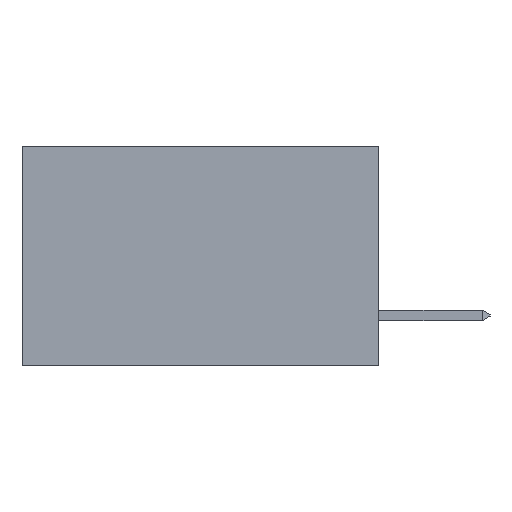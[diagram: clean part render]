
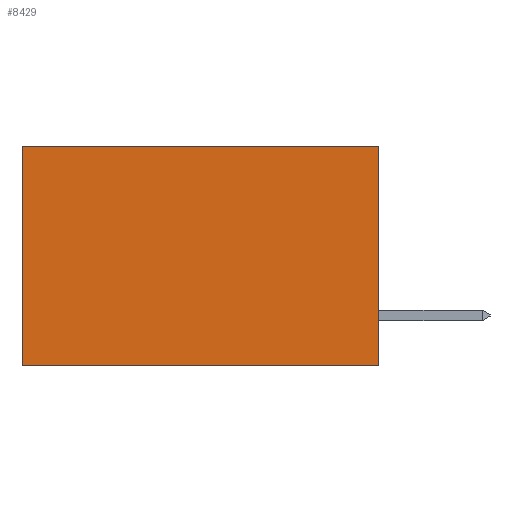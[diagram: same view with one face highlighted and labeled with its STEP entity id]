
A CAD part, left-side view. The second image highlights one B-rep face of the part: STEP entity #8429.
In plain terms, the highlighted planar face has unit normal (-1, 0, 0).
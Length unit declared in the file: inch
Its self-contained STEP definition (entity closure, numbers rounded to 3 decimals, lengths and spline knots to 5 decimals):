
#225 = PLANE ( 'NONE',  #2676 ) ;
#362 = CARTESIAN_POINT ( 'NONE',  ( 0.298, 0., 0. ) ) ;
#489 = CARTESIAN_POINT ( 'NONE',  ( 0.298, 0.6, 0. ) ) ;
#917 = VERTEX_POINT ( 'NONE', #10837 ) ;
#1516 = ORIENTED_EDGE ( 'NONE', *, *, #3124, .F. ) ;
#2676 = AXIS2_PLACEMENT_3D ( 'NONE', #362, #3206, #3161 ) ;
#2751 = CARTESIAN_POINT ( 'NONE',  ( 0.298, 0., 0. ) ) ;
#3083 = EDGE_CURVE ( 'NONE', #8026, #4044, #15981, .T. ) ;
#3124 = EDGE_CURVE ( 'NONE', #3225, #917, #15474, .T. ) ;
#3145 = LINE ( 'NONE', #2751, #19658 ) ;
#3161 = DIRECTION ( 'NONE',  ( 0., 0., -1. ) ) ;
#3206 = DIRECTION ( 'NONE',  ( 1., 0., 0. ) ) ;
#3225 = VERTEX_POINT ( 'NONE', #13918 ) ;
#3390 = ORIENTED_EDGE ( 'NONE', *, *, #3083, .T. ) ;
#3774 = EDGE_LOOP ( 'NONE', ( #3390, #14959, #1516, #17273 ) ) ;
#4044 = VERTEX_POINT ( 'NONE', #15296 ) ;
#6623 = VECTOR ( 'NONE', #13806, 39.37008 ) ;
#7162 = VECTOR ( 'NONE', #12559, 39.37008 ) ;
#7775 = DIRECTION ( 'NONE',  ( 0., 1., 0. ) ) ;
#8026 = VERTEX_POINT ( 'NONE', #489 ) ;
#8429 = ADVANCED_FACE ( 'NONE', ( #15243 ), #225, .F. ) ;
#10480 = LINE ( 'NONE', #10987, #18141 ) ;
#10837 = CARTESIAN_POINT ( 'NONE',  ( 0.298, 0., -0.37 ) ) ;
#10987 = CARTESIAN_POINT ( 'NONE',  ( 0.298, 0., -0.37 ) ) ;
#11454 = EDGE_CURVE ( 'NONE', #917, #4044, #10480, .T. ) ;
#11765 = CARTESIAN_POINT ( 'NONE',  ( 0.298, 0., 0. ) ) ;
#12559 = DIRECTION ( 'NONE',  ( 0., 0., -1. ) ) ;
#12664 = DIRECTION ( 'NONE',  ( 0., 1., 0. ) ) ;
#13806 = DIRECTION ( 'NONE',  ( 0., 0., -1. ) ) ;
#13918 = CARTESIAN_POINT ( 'NONE',  ( 0.298, 0., 0. ) ) ;
#14959 = ORIENTED_EDGE ( 'NONE', *, *, #11454, .F. ) ;
#15243 = FACE_OUTER_BOUND ( 'NONE', #3774, .T. ) ;
#15296 = CARTESIAN_POINT ( 'NONE',  ( 0.298, 0.6, -0.37 ) ) ;
#15474 = LINE ( 'NONE', #11765, #6623 ) ;
#15981 = LINE ( 'NONE', #19376, #7162 ) ;
#17273 = ORIENTED_EDGE ( 'NONE', *, *, #21156, .T. ) ;
#18141 = VECTOR ( 'NONE', #12664, 39.37008 ) ;
#19376 = CARTESIAN_POINT ( 'NONE',  ( 0.298, 0.6, 0. ) ) ;
#19658 = VECTOR ( 'NONE', #7775, 39.37008 ) ;
#21156 = EDGE_CURVE ( 'NONE', #3225, #8026, #3145, .T. ) ;
